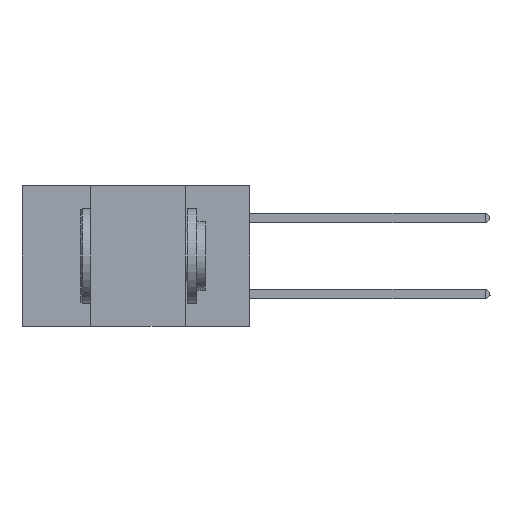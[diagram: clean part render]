
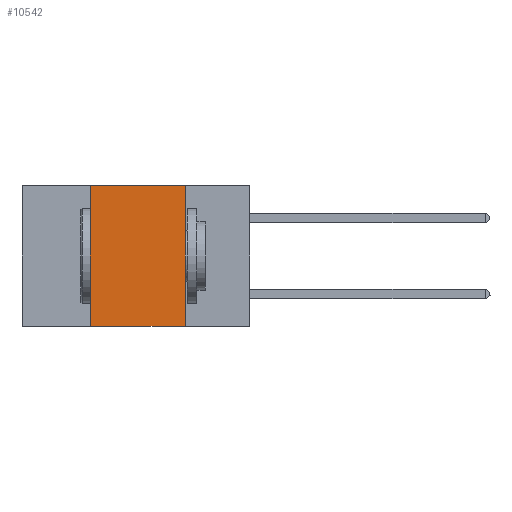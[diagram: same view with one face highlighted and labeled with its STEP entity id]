
A CAD part, left-side view. The second image highlights one B-rep face of the part: STEP entity #10542.
In plain terms, the highlighted planar face has unit normal (-1, 0, 0).
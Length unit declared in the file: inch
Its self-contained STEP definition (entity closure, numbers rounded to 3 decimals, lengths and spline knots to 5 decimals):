
#219 = ORIENTED_EDGE ( 'NONE', *, *, #829, .T. ) ;
#283 = EDGE_LOOP ( 'NONE', ( #15430, #10982, #7065, #219 ) ) ;
#829 = EDGE_CURVE ( 'NONE', #12641, #15021, #12533, .T. ) ;
#1002 = EDGE_CURVE ( 'NONE', #9142, #5237, #12991, .T. ) ;
#1631 = CARTESIAN_POINT ( 'NONE',  ( 0., 0.17, 0. ) ) ;
#3305 = DIRECTION ( 'NONE',  ( 0., -1., 0. ) ) ;
#3679 = VECTOR ( 'NONE', #9158, 39.37008 ) ;
#4333 = CARTESIAN_POINT ( 'NONE',  ( 0., 0.17, -0.37 ) ) ;
#4533 = CARTESIAN_POINT ( 'NONE',  ( 0., 0.6, 0. ) ) ;
#4585 = CARTESIAN_POINT ( 'NONE',  ( 0., 0.17, 0. ) ) ;
#5237 = VERTEX_POINT ( 'NONE', #4585 ) ;
#6106 = EDGE_CURVE ( 'NONE', #12641, #9142, #15331, .T. ) ;
#6256 = CARTESIAN_POINT ( 'NONE',  ( 0., 0.42, 0. ) ) ;
#7065 = ORIENTED_EDGE ( 'NONE', *, *, #6106, .F. ) ;
#7620 = DIRECTION ( 'NONE',  ( 0., 0., -1. ) ) ;
#8044 = DIRECTION ( 'NONE',  ( 0., -1., 0. ) ) ;
#9142 = VERTEX_POINT ( 'NONE', #18089 ) ;
#9158 = DIRECTION ( 'NONE',  ( 0., 0., 1. ) ) ;
#10542 = ADVANCED_FACE ( 'NONE', ( #14295 ), #14627, .F. ) ;
#10982 = ORIENTED_EDGE ( 'NONE', *, *, #1002, .F. ) ;
#11312 = CARTESIAN_POINT ( 'NONE',  ( 0., 0.42, -0.37 ) ) ;
#11627 = DIRECTION ( 'NONE',  ( 0., 0., -1. ) ) ;
#12216 = LINE ( 'NONE', #1631, #17269 ) ;
#12533 = LINE ( 'NONE', #13698, #13407 ) ;
#12641 = VERTEX_POINT ( 'NONE', #11312 ) ;
#12991 = LINE ( 'NONE', #4533, #13636 ) ;
#13209 = CARTESIAN_POINT ( 'NONE',  ( 0., 0.6, 0. ) ) ;
#13407 = VECTOR ( 'NONE', #8044, 39.37008 ) ;
#13636 = VECTOR ( 'NONE', #3305, 39.37008 ) ;
#13698 = CARTESIAN_POINT ( 'NONE',  ( 0., 0.6, -0.37 ) ) ;
#14295 = FACE_OUTER_BOUND ( 'NONE', #283, .T. ) ;
#14627 = PLANE ( 'NONE',  #17253 ) ;
#15021 = VERTEX_POINT ( 'NONE', #4333 ) ;
#15331 = LINE ( 'NONE', #6256, #3679 ) ;
#15430 = ORIENTED_EDGE ( 'NONE', *, *, #17504, .F. ) ;
#16034 = DIRECTION ( 'NONE',  ( 1., 0., 0. ) ) ;
#17253 = AXIS2_PLACEMENT_3D ( 'NONE', #13209, #16034, #7620 ) ;
#17269 = VECTOR ( 'NONE', #11627, 39.37008 ) ;
#17504 = EDGE_CURVE ( 'NONE', #5237, #15021, #12216, .T. ) ;
#18089 = CARTESIAN_POINT ( 'NONE',  ( 0., 0.42, 0. ) ) ;
